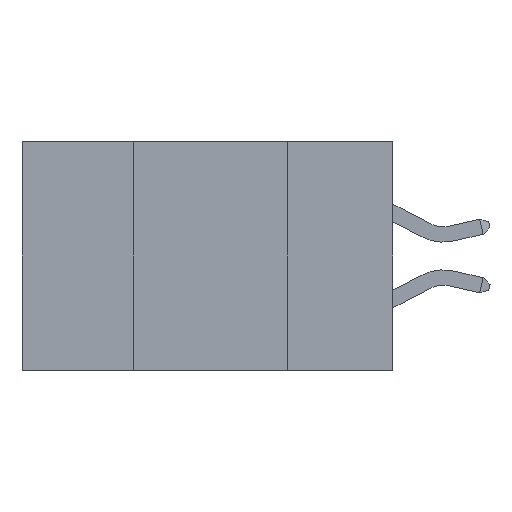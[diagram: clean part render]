
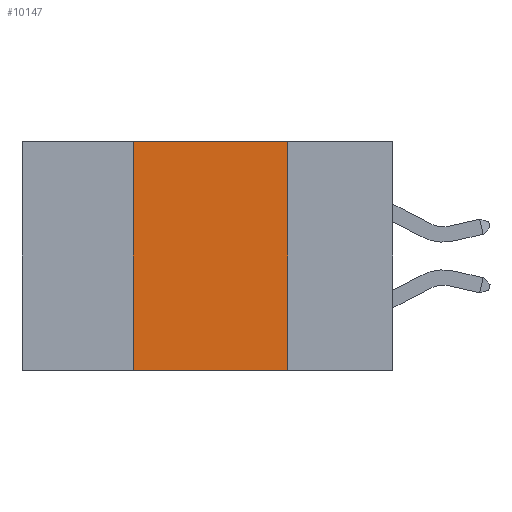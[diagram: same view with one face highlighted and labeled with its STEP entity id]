
A CAD part, left-side view. The second image highlights one B-rep face of the part: STEP entity #10147.
In plain terms, the highlighted planar face has unit normal (-1, 0, 0).
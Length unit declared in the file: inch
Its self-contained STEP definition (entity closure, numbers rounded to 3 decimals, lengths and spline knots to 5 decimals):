
#6 = EDGE_CURVE ( 'NONE', #4463, #10058, #6596, .T. ) ;
#1473 = CARTESIAN_POINT ( 'NONE',  ( 0., 0.42, 0. ) ) ;
#1819 = LINE ( 'NONE', #2078, #4270 ) ;
#1912 = CARTESIAN_POINT ( 'NONE',  ( 0., 0.6, -0.37 ) ) ;
#1965 = DIRECTION ( 'NONE',  ( 0., 0., -1. ) ) ;
#2033 = VECTOR ( 'NONE', #1965, 39.37008 ) ;
#2078 = CARTESIAN_POINT ( 'NONE',  ( 0., 0.6, 0. ) ) ;
#2100 = EDGE_CURVE ( 'NONE', #10058, #2964, #1819, .T. ) ;
#2168 = LINE ( 'NONE', #7662, #2033 ) ;
#2233 = ORIENTED_EDGE ( 'NONE', *, *, #4962, .F. ) ;
#2964 = VERTEX_POINT ( 'NONE', #3355 ) ;
#3355 = CARTESIAN_POINT ( 'NONE',  ( 0., 0.17, 0. ) ) ;
#3710 = ORIENTED_EDGE ( 'NONE', *, *, #2100, .F. ) ;
#3725 = DIRECTION ( 'NONE',  ( 0., -1., 0. ) ) ;
#3855 = FACE_OUTER_BOUND ( 'NONE', #4513, .T. ) ;
#4270 = VECTOR ( 'NONE', #3725, 39.37008 ) ;
#4463 = VERTEX_POINT ( 'NONE', #4545 ) ;
#4513 = EDGE_LOOP ( 'NONE', ( #2233, #3710, #6434, #5798 ) ) ;
#4545 = CARTESIAN_POINT ( 'NONE',  ( 0., 0.42, -0.37 ) ) ;
#4962 = EDGE_CURVE ( 'NONE', #2964, #6606, #2168, .T. ) ;
#5016 = AXIS2_PLACEMENT_3D ( 'NONE', #7294, #7326, #8189 ) ;
#5468 = CARTESIAN_POINT ( 'NONE',  ( 0., 0.42, 0. ) ) ;
#5535 = LINE ( 'NONE', #1912, #8733 ) ;
#5798 = ORIENTED_EDGE ( 'NONE', *, *, #8767, .T. ) ;
#6434 = ORIENTED_EDGE ( 'NONE', *, *, #6, .F. ) ;
#6596 = LINE ( 'NONE', #1473, #8399 ) ;
#6606 = VERTEX_POINT ( 'NONE', #7069 ) ;
#7069 = CARTESIAN_POINT ( 'NONE',  ( 0., 0.17, -0.37 ) ) ;
#7294 = CARTESIAN_POINT ( 'NONE',  ( 0., 0.6, 0. ) ) ;
#7326 = DIRECTION ( 'NONE',  ( 1., 0., 0. ) ) ;
#7395 = PLANE ( 'NONE',  #5016 ) ;
#7662 = CARTESIAN_POINT ( 'NONE',  ( 0., 0.17, 0. ) ) ;
#8189 = DIRECTION ( 'NONE',  ( 0., 0., -1. ) ) ;
#8399 = VECTOR ( 'NONE', #10443, 39.37008 ) ;
#8541 = DIRECTION ( 'NONE',  ( 0., -1., 0. ) ) ;
#8733 = VECTOR ( 'NONE', #8541, 39.37008 ) ;
#8767 = EDGE_CURVE ( 'NONE', #4463, #6606, #5535, .T. ) ;
#10058 = VERTEX_POINT ( 'NONE', #5468 ) ;
#10147 = ADVANCED_FACE ( 'NONE', ( #3855 ), #7395, .F. ) ;
#10443 = DIRECTION ( 'NONE',  ( 0., 0., 1. ) ) ;
